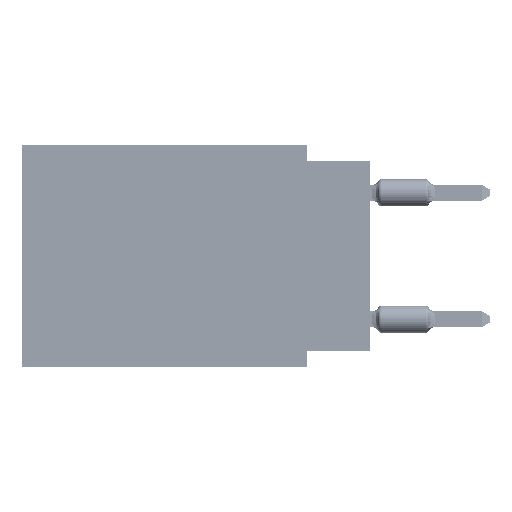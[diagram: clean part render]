
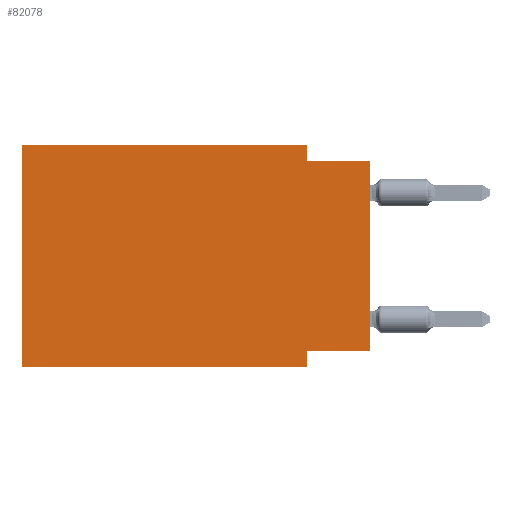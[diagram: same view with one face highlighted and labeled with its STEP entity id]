
A CAD part, left-side view. The second image highlights one B-rep face of the part: STEP entity #82078.
In plain terms, the highlighted planar face has unit normal (-1, 0, 0).
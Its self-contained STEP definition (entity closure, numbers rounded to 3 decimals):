
#161 = EDGE_CURVE ( 'NONE', #70919, #28368, #18596, .T. ) ;
#648 = EDGE_CURVE ( 'NONE', #88255, #20929, #75663, .T. ) ;
#1609 = VERTEX_POINT ( 'NONE', #73885 ) ;
#2573 = DIRECTION ( 'NONE',  ( 0., 0., 1. ) ) ;
#2828 = VECTOR ( 'NONE', #29766, 1000. ) ;
#2990 = VECTOR ( 'NONE', #101234, 1000. ) ;
#12489 = LINE ( 'NONE', #30004, #40905 ) ;
#12846 = VERTEX_POINT ( 'NONE', #78925 ) ;
#14020 = VECTOR ( 'NONE', #82382, 1000. ) ;
#14091 = DIRECTION ( 'NONE',  ( 1., 0., 0. ) ) ;
#14707 = ORIENTED_EDGE ( 'NONE', *, *, #69515, .F. ) ;
#15901 = EDGE_CURVE ( 'NONE', #12846, #20929, #95925, .T. ) ;
#16181 = ORIENTED_EDGE ( 'NONE', *, *, #43969, .T. ) ;
#17254 = ORIENTED_EDGE ( 'NONE', *, *, #648, .F. ) ;
#18596 = LINE ( 'NONE', #50047, #76561 ) ;
#20792 = CARTESIAN_POINT ( 'NONE',  ( 0., 13.97, 0. ) ) ;
#20929 = VERTEX_POINT ( 'NONE', #46483 ) ;
#21764 = DIRECTION ( 'NONE',  ( 0., -1., 0. ) ) ;
#25527 = CARTESIAN_POINT ( 'NONE',  ( 0., 2.54, -8.89 ) ) ;
#28368 = VERTEX_POINT ( 'NONE', #25527 ) ;
#29391 = EDGE_CURVE ( 'NONE', #12846, #70919, #78664, .T. ) ;
#29766 = DIRECTION ( 'NONE',  ( 0., 1., 0. ) ) ;
#30004 = CARTESIAN_POINT ( 'NONE',  ( 0., 13.97, 0. ) ) ;
#32741 = ORIENTED_EDGE ( 'NONE', *, *, #45500, .F. ) ;
#38346 = LINE ( 'NONE', #69764, #2990 ) ;
#38388 = DIRECTION ( 'NONE',  ( 0., 0., -1. ) ) ;
#39652 = CARTESIAN_POINT ( 'NONE',  ( 0., 13.97, 0. ) ) ;
#40905 = VECTOR ( 'NONE', #21764, 1000. ) ;
#41271 = CARTESIAN_POINT ( 'NONE',  ( 0., 2.54, 0. ) ) ;
#41505 = AXIS2_PLACEMENT_3D ( 'NONE', #20792, #14091, #99672 ) ;
#41787 = CARTESIAN_POINT ( 'NONE',  ( 0., 0., 0. ) ) ;
#43969 = EDGE_CURVE ( 'NONE', #1609, #28368, #38346, .T. ) ;
#45035 = PLANE ( 'NONE',  #41505 ) ;
#45500 = EDGE_CURVE ( 'NONE', #80621, #92080, #12489, .T. ) ;
#46483 = CARTESIAN_POINT ( 'NONE',  ( 0., 0., -0.635 ) ) ;
#50047 = CARTESIAN_POINT ( 'NONE',  ( 0., 2.54, -8.89 ) ) ;
#56152 = DIRECTION ( 'NONE',  ( 0., 0., 1. ) ) ;
#58586 = EDGE_CURVE ( 'NONE', #92080, #88255, #73864, .T. ) ;
#64611 = CARTESIAN_POINT ( 'NONE',  ( 0., 2.54, 0. ) ) ;
#69373 = ORIENTED_EDGE ( 'NONE', *, *, #161, .F. ) ;
#69515 = EDGE_CURVE ( 'NONE', #1609, #80621, #71581, .T. ) ;
#69764 = CARTESIAN_POINT ( 'NONE',  ( 0., 13.97, -8.89 ) ) ;
#70919 = VERTEX_POINT ( 'NONE', #92115 ) ;
#71581 = LINE ( 'NONE', #77806, #88291 ) ;
#73864 = LINE ( 'NONE', #64611, #85359 ) ;
#73885 = CARTESIAN_POINT ( 'NONE',  ( 0., 13.97, -8.89 ) ) ;
#74126 = VECTOR ( 'NONE', #2573, 1000. ) ;
#74127 = CARTESIAN_POINT ( 'NONE',  ( 0., 0., -0.635 ) ) ;
#75663 = LINE ( 'NONE', #74127, #14020 ) ;
#76561 = VECTOR ( 'NONE', #38388, 1000. ) ;
#77806 = CARTESIAN_POINT ( 'NONE',  ( 0., 13.97, 0. ) ) ;
#78664 = LINE ( 'NONE', #100393, #2828 ) ;
#78925 = CARTESIAN_POINT ( 'NONE',  ( 0., 0., -8.255 ) ) ;
#80009 = CARTESIAN_POINT ( 'NONE',  ( 0., 2.54, -0.635 ) ) ;
#80621 = VERTEX_POINT ( 'NONE', #39652 ) ;
#82078 = ADVANCED_FACE ( 'NONE', ( #84709 ), #45035, .F. ) ;
#82382 = DIRECTION ( 'NONE',  ( 0., -1., 0. ) ) ;
#84709 = FACE_OUTER_BOUND ( 'NONE', #86306, .T. ) ;
#85359 = VECTOR ( 'NONE', #89352, 1000. ) ;
#86306 = EDGE_LOOP ( 'NONE', ( #95344, #17254, #93957, #32741, #14707, #16181, #69373, #89297 ) ) ;
#88255 = VERTEX_POINT ( 'NONE', #80009 ) ;
#88291 = VECTOR ( 'NONE', #56152, 1000. ) ;
#89297 = ORIENTED_EDGE ( 'NONE', *, *, #29391, .F. ) ;
#89352 = DIRECTION ( 'NONE',  ( 0., 0., -1. ) ) ;
#92080 = VERTEX_POINT ( 'NONE', #41271 ) ;
#92115 = CARTESIAN_POINT ( 'NONE',  ( 0., 2.54, -8.255 ) ) ;
#93957 = ORIENTED_EDGE ( 'NONE', *, *, #58586, .F. ) ;
#95344 = ORIENTED_EDGE ( 'NONE', *, *, #15901, .T. ) ;
#95925 = LINE ( 'NONE', #41787, #74126 ) ;
#99672 = DIRECTION ( 'NONE',  ( 0., 0., -1. ) ) ;
#100393 = CARTESIAN_POINT ( 'NONE',  ( 0., 0., -8.255 ) ) ;
#101234 = DIRECTION ( 'NONE',  ( 0., -1., 0. ) ) ;
